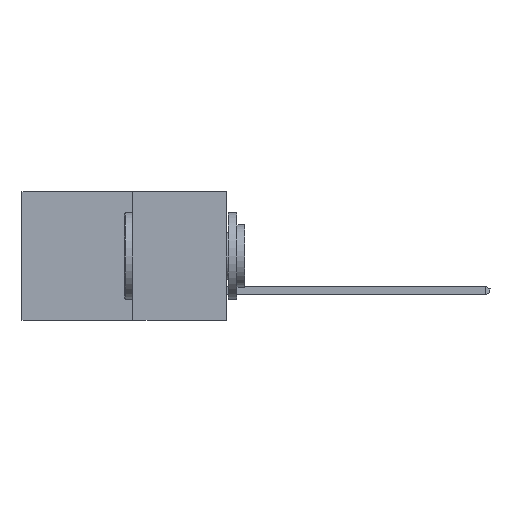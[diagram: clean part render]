
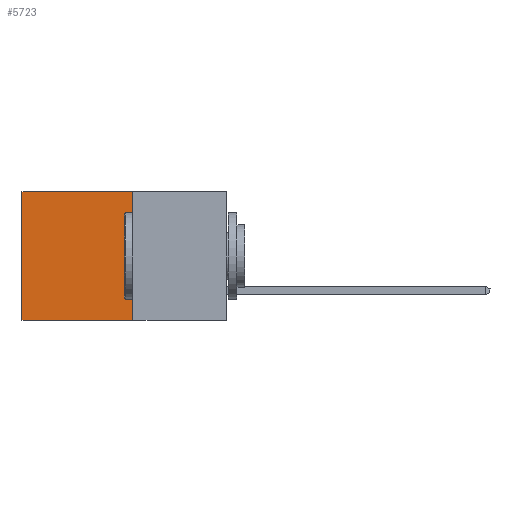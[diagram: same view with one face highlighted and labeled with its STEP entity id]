
A CAD part, left-side view. The second image highlights one B-rep face of the part: STEP entity #5723.
In plain terms, the highlighted planar face has unit normal (-1, 0, 0).
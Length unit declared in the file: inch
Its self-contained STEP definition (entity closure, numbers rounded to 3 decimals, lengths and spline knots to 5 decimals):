
#213 = EDGE_CURVE ( 'NONE', #11434, #1597, #6519, .T. ) ;
#444 = CARTESIAN_POINT ( 'NONE',  ( 0.277, 0.27, -0.37 ) ) ;
#773 = VECTOR ( 'NONE', #7841, 39.37008 ) ;
#1502 = CARTESIAN_POINT ( 'NONE',  ( 0.277, 0.59, -0.37 ) ) ;
#1597 = VERTEX_POINT ( 'NONE', #13186 ) ;
#1747 = CARTESIAN_POINT ( 'NONE',  ( 0.277, 0.27, -0.37 ) ) ;
#2033 = EDGE_LOOP ( 'NONE', ( #3918, #6879, #12573, #10094 ) ) ;
#2342 = LINE ( 'NONE', #13684, #4918 ) ;
#2905 = DIRECTION ( 'NONE',  ( 0., 1., 0. ) ) ;
#3918 = ORIENTED_EDGE ( 'NONE', *, *, #7662, .T. ) ;
#3982 = AXIS2_PLACEMENT_3D ( 'NONE', #444, #11379, #11341 ) ;
#4918 = VECTOR ( 'NONE', #2905, 39.37008 ) ;
#5463 = CARTESIAN_POINT ( 'NONE',  ( 0.277, 0.27, -0.37 ) ) ;
#5604 = VECTOR ( 'NONE', #12645, 39.37008 ) ;
#5723 = ADVANCED_FACE ( 'NONE', ( #13611 ), #11358, .F. ) ;
#6519 = LINE ( 'NONE', #10271, #11893 ) ;
#6716 = LINE ( 'NONE', #7832, #773 ) ;
#6879 = ORIENTED_EDGE ( 'NONE', *, *, #10266, .F. ) ;
#7662 = EDGE_CURVE ( 'NONE', #1597, #10812, #6716, .T. ) ;
#7832 = CARTESIAN_POINT ( 'NONE',  ( 0.277, 0.59, -0.37 ) ) ;
#7841 = DIRECTION ( 'NONE',  ( 0., 0., -1. ) ) ;
#8253 = DIRECTION ( 'NONE',  ( 0., 1., 0. ) ) ;
#8968 = EDGE_CURVE ( 'NONE', #11434, #9143, #14175, .T. ) ;
#9143 = VERTEX_POINT ( 'NONE', #5463 ) ;
#10094 = ORIENTED_EDGE ( 'NONE', *, *, #213, .T. ) ;
#10266 = EDGE_CURVE ( 'NONE', #9143, #10812, #2342, .T. ) ;
#10271 = CARTESIAN_POINT ( 'NONE',  ( 0.277, 0.27, 0. ) ) ;
#10285 = CARTESIAN_POINT ( 'NONE',  ( 0.277, 0.27, 0. ) ) ;
#10812 = VERTEX_POINT ( 'NONE', #1502 ) ;
#11341 = DIRECTION ( 'NONE',  ( 0., 0., -1. ) ) ;
#11358 = PLANE ( 'NONE',  #3982 ) ;
#11379 = DIRECTION ( 'NONE',  ( 1., 0., 0. ) ) ;
#11434 = VERTEX_POINT ( 'NONE', #10285 ) ;
#11893 = VECTOR ( 'NONE', #8253, 39.37008 ) ;
#12573 = ORIENTED_EDGE ( 'NONE', *, *, #8968, .F. ) ;
#12645 = DIRECTION ( 'NONE',  ( 0., 0., -1. ) ) ;
#13186 = CARTESIAN_POINT ( 'NONE',  ( 0.277, 0.59, 0. ) ) ;
#13611 = FACE_OUTER_BOUND ( 'NONE', #2033, .T. ) ;
#13684 = CARTESIAN_POINT ( 'NONE',  ( 0.277, 0.27, -0.37 ) ) ;
#14175 = LINE ( 'NONE', #1747, #5604 ) ;
